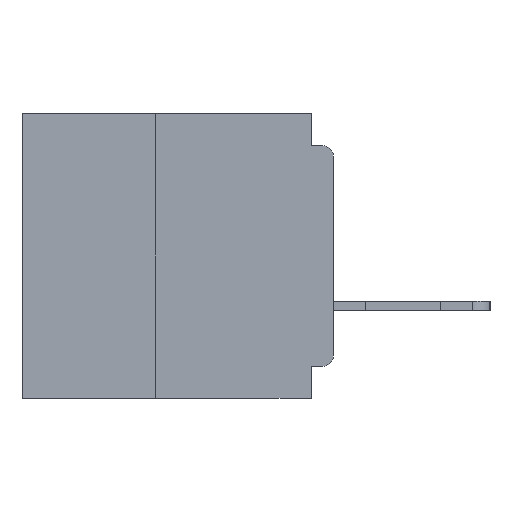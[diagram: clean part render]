
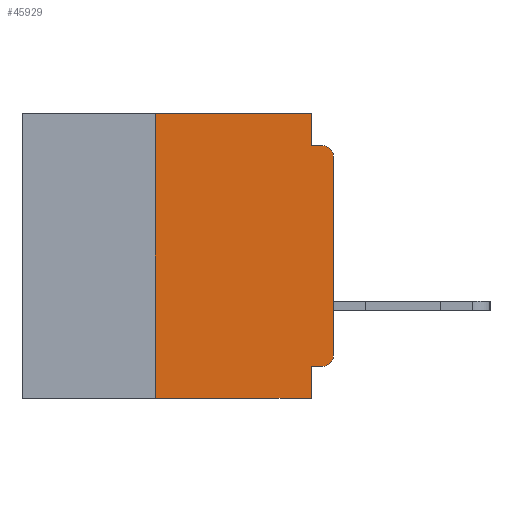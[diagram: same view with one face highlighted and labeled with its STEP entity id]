
A CAD part, left-side view. The second image highlights one B-rep face of the part: STEP entity #45929.
In plain terms, the highlighted planar face has unit normal (-1, 0, 0).
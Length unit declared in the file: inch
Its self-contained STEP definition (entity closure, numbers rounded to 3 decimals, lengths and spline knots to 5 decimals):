
#220 = VECTOR ( 'NONE', #10136, 39.37008 ) ;
#333 = ORIENTED_EDGE ( 'NONE', *, *, #18744, .F. ) ;
#575 = EDGE_CURVE ( 'NONE', #20642, #2816, #19092, .T. ) ;
#1032 = FACE_OUTER_BOUND ( 'NONE', #48521, .T. ) ;
#1259 = DIRECTION ( 'NONE',  ( 0., -1., 0. ) ) ;
#1278 = VERTEX_POINT ( 'NONE', #20155 ) ;
#1523 = EDGE_CURVE ( 'NONE', #19784, #20642, #7858, .T. ) ;
#1771 = CARTESIAN_POINT ( 'NONE',  ( 0., 0.437, 0. ) ) ;
#2295 = CARTESIAN_POINT ( 'NONE',  ( 0., 0., -0.355 ) ) ;
#2399 = EDGE_CURVE ( 'NONE', #2816, #1278, #28302, .T. ) ;
#2816 = VERTEX_POINT ( 'NONE', #33389 ) ;
#3745 = PLANE ( 'NONE',  #42046 ) ;
#4836 = EDGE_CURVE ( 'NONE', #1278, #21661, #44396, .T. ) ;
#5952 = DIRECTION ( 'NONE',  ( -1., 0., 0. ) ) ;
#6988 = CARTESIAN_POINT ( 'NONE',  ( 0., 0., -0.045 ) ) ;
#7425 = ORIENTED_EDGE ( 'NONE', *, *, #2399, .F. ) ;
#7858 = LINE ( 'NONE', #47613, #220 ) ;
#9118 = VECTOR ( 'NONE', #1259, 39.37008 ) ;
#9987 = CIRCLE ( 'NONE', #35233, 0.015 ) ;
#10136 = DIRECTION ( 'NONE',  ( 0., 0., 1. ) ) ;
#10625 = VECTOR ( 'NONE', #37614, 39.37008 ) ;
#11250 = ORIENTED_EDGE ( 'NONE', *, *, #575, .F. ) ;
#11375 = CARTESIAN_POINT ( 'NONE',  ( 0., 0.015, -0.06 ) ) ;
#12894 = VECTOR ( 'NONE', #18208, 39.37008 ) ;
#13010 = VERTEX_POINT ( 'NONE', #21446 ) ;
#14488 = VERTEX_POINT ( 'NONE', #42309 ) ;
#15032 = DIRECTION ( 'NONE',  ( 1., 0., 0. ) ) ;
#15052 = DIRECTION ( 'NONE',  ( 0., 0., 1. ) ) ;
#15159 = DIRECTION ( 'NONE',  ( 0., 0., -1. ) ) ;
#16370 = LINE ( 'NONE', #2295, #27435 ) ;
#17232 = VECTOR ( 'NONE', #41680, 39.37008 ) ;
#17538 = VERTEX_POINT ( 'NONE', #37153 ) ;
#18052 = ORIENTED_EDGE ( 'NONE', *, *, #1523, .F. ) ;
#18208 = DIRECTION ( 'NONE',  ( 0., 0., -1. ) ) ;
#18293 = DIRECTION ( 'NONE',  ( 0., -1., 0. ) ) ;
#18397 = EDGE_CURVE ( 'NONE', #14488, #45436, #35083, .T. ) ;
#18744 = EDGE_CURVE ( 'NONE', #17538, #14488, #16370, .T. ) ;
#19076 = CARTESIAN_POINT ( 'NONE',  ( 0., 0.031, 0. ) ) ;
#19092 = LINE ( 'NONE', #1771, #9118 ) ;
#19382 = CARTESIAN_POINT ( 'NONE',  ( 0., 0.015, -0.045 ) ) ;
#19784 = VERTEX_POINT ( 'NONE', #30638 ) ;
#20155 = CARTESIAN_POINT ( 'NONE',  ( 0., 0.031, -0.045 ) ) ;
#20523 = AXIS2_PLACEMENT_3D ( 'NONE', #28333, #5952, #32117 ) ;
#20642 = VERTEX_POINT ( 'NONE', #39621 ) ;
#21446 = CARTESIAN_POINT ( 'NONE',  ( 0., 0., -0.34 ) ) ;
#21661 = VERTEX_POINT ( 'NONE', #19382 ) ;
#22665 = EDGE_CURVE ( 'NONE', #13010, #36492, #33168, .T. ) ;
#23215 = VECTOR ( 'NONE', #15052, 39.37008 ) ;
#24136 = ORIENTED_EDGE ( 'NONE', *, *, #40547, .T. ) ;
#26126 = DIRECTION ( 'NONE',  ( 0., 0., -1. ) ) ;
#27435 = VECTOR ( 'NONE', #28433, 39.37008 ) ;
#28036 = ORIENTED_EDGE ( 'NONE', *, *, #4836, .F. ) ;
#28208 = CIRCLE ( 'NONE', #20523, 0.015 ) ;
#28302 = LINE ( 'NONE', #19076, #17232 ) ;
#28333 = CARTESIAN_POINT ( 'NONE',  ( 0., 0.015, -0.34 ) ) ;
#28433 = DIRECTION ( 'NONE',  ( 0., 1., 0. ) ) ;
#29050 = CARTESIAN_POINT ( 'NONE',  ( 0., 0., -0.06 ) ) ;
#29417 = ORIENTED_EDGE ( 'NONE', *, *, #34185, .T. ) ;
#30052 = CARTESIAN_POINT ( 'NONE',  ( 0., 0., 0. ) ) ;
#30638 = CARTESIAN_POINT ( 'NONE',  ( 0., 0.25, -0.4 ) ) ;
#31577 = ORIENTED_EDGE ( 'NONE', *, *, #39468, .T. ) ;
#32117 = DIRECTION ( 'NONE',  ( 0., 0., -1. ) ) ;
#33168 = LINE ( 'NONE', #30052, #23215 ) ;
#33389 = CARTESIAN_POINT ( 'NONE',  ( 0., 0.031, 0. ) ) ;
#33830 = CARTESIAN_POINT ( 'NONE',  ( 0., 0.437, -0.4 ) ) ;
#34185 = EDGE_CURVE ( 'NONE', #19784, #45436, #40544, .T. ) ;
#34372 = VECTOR ( 'NONE', #18293, 39.37008 ) ;
#34456 = ORIENTED_EDGE ( 'NONE', *, *, #22665, .T. ) ;
#35083 = LINE ( 'NONE', #36826, #12894 ) ;
#35233 = AXIS2_PLACEMENT_3D ( 'NONE', #11375, #37555, #15159 ) ;
#36492 = VERTEX_POINT ( 'NONE', #29050 ) ;
#36826 = CARTESIAN_POINT ( 'NONE',  ( 0., 0.031, -0.4 ) ) ;
#37153 = CARTESIAN_POINT ( 'NONE',  ( 0., 0.015, -0.355 ) ) ;
#37269 = CARTESIAN_POINT ( 'NONE',  ( 0., 0.437, 0. ) ) ;
#37555 = DIRECTION ( 'NONE',  ( -1., 0., 0. ) ) ;
#37614 = DIRECTION ( 'NONE',  ( 0., -1., 0. ) ) ;
#37977 = CARTESIAN_POINT ( 'NONE',  ( 0., 0.031, -0.4 ) ) ;
#39468 = EDGE_CURVE ( 'NONE', #17538, #13010, #28208, .T. ) ;
#39621 = CARTESIAN_POINT ( 'NONE',  ( 0., 0.25, 0. ) ) ;
#40544 = LINE ( 'NONE', #33830, #10625 ) ;
#40547 = EDGE_CURVE ( 'NONE', #36492, #21661, #9987, .T. ) ;
#41279 = ORIENTED_EDGE ( 'NONE', *, *, #18397, .F. ) ;
#41680 = DIRECTION ( 'NONE',  ( 0., 0., -1. ) ) ;
#42046 = AXIS2_PLACEMENT_3D ( 'NONE', #37269, #15032, #26126 ) ;
#42309 = CARTESIAN_POINT ( 'NONE',  ( 0., 0.031, -0.355 ) ) ;
#44396 = LINE ( 'NONE', #6988, #34372 ) ;
#45436 = VERTEX_POINT ( 'NONE', #37977 ) ;
#45929 = ADVANCED_FACE ( 'NONE', ( #1032 ), #3745, .F. ) ;
#47613 = CARTESIAN_POINT ( 'NONE',  ( 0., 0.25, -0.4 ) ) ;
#48521 = EDGE_LOOP ( 'NONE', ( #34456, #24136, #28036, #7425, #11250, #18052, #29417, #41279, #333, #31577 ) ) ;
